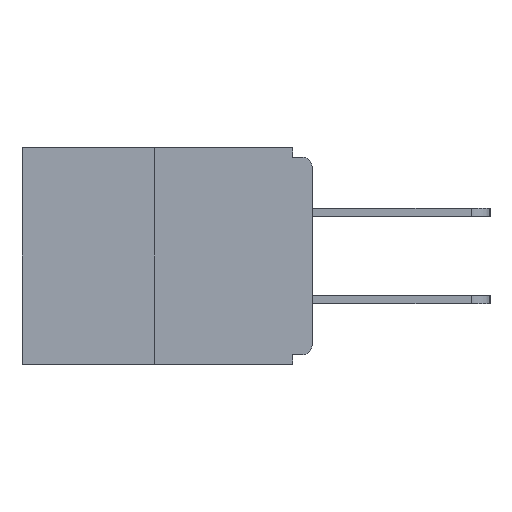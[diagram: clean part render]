
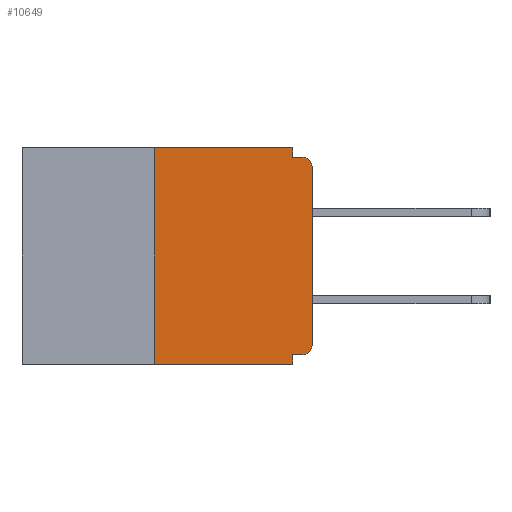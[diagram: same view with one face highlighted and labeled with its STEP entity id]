
A CAD part, left-side view. The second image highlights one B-rep face of the part: STEP entity #10649.
In plain terms, the highlighted planar face has unit normal (-1, 0, 0).
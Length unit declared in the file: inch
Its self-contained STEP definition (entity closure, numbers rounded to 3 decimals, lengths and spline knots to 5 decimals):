
#17 = CARTESIAN_POINT ( 'NONE',  ( 0., 0.015, -0.328 ) ) ;
#86 = ORIENTED_EDGE ( 'NONE', *, *, #10237, .F. ) ;
#189 = VERTEX_POINT ( 'NONE', #1568 ) ;
#205 = LINE ( 'NONE', #12582, #10612 ) ;
#230 = LINE ( 'NONE', #5191, #6545 ) ;
#375 = LINE ( 'NONE', #4759, #1457 ) ;
#461 = EDGE_CURVE ( 'NONE', #4245, #189, #2038, .T. ) ;
#812 = DIRECTION ( 'NONE',  ( 0., 0., -1. ) ) ;
#832 = DIRECTION ( 'NONE',  ( -1., 0., 0. ) ) ;
#939 = VERTEX_POINT ( 'NONE', #12508 ) ;
#1054 = DIRECTION ( 'NONE',  ( 0., -1., 0. ) ) ;
#1457 = VECTOR ( 'NONE', #12794, 39.37008 ) ;
#1568 = CARTESIAN_POINT ( 'NONE',  ( 0., 0.015, -0.015 ) ) ;
#1638 = DIRECTION ( 'NONE',  ( 0., 0., 1. ) ) ;
#1753 = CARTESIAN_POINT ( 'NONE',  ( 0., 0.015, -0.313 ) ) ;
#1868 = DIRECTION ( 'NONE',  ( 0., 1., 0. ) ) ;
#2038 = CIRCLE ( 'NONE', #5717, 0.015 ) ;
#2332 = VECTOR ( 'NONE', #4562, 39.37008 ) ;
#2425 = AXIS2_PLACEMENT_3D ( 'NONE', #1753, #832, #7921 ) ;
#2665 = ORIENTED_EDGE ( 'NONE', *, *, #10603, .T. ) ;
#2852 = LINE ( 'NONE', #7215, #5706 ) ;
#3024 = DIRECTION ( 'NONE',  ( 0., 0., -1. ) ) ;
#3090 = ORIENTED_EDGE ( 'NONE', *, *, #461, .T. ) ;
#3254 = CARTESIAN_POINT ( 'NONE',  ( 0., 0.031, 0. ) ) ;
#3560 = EDGE_CURVE ( 'NONE', #5918, #189, #230, .T. ) ;
#4131 = EDGE_CURVE ( 'NONE', #10853, #5918, #6677, .T. ) ;
#4152 = EDGE_CURVE ( 'NONE', #7958, #7381, #6830, .T. ) ;
#4245 = VERTEX_POINT ( 'NONE', #6832 ) ;
#4494 = ORIENTED_EDGE ( 'NONE', *, *, #7804, .F. ) ;
#4562 = DIRECTION ( 'NONE',  ( 0., -1., 0. ) ) ;
#4749 = EDGE_CURVE ( 'NONE', #10086, #7619, #205, .T. ) ;
#4759 = CARTESIAN_POINT ( 'NONE',  ( 0., 0.031, -0.343 ) ) ;
#4770 = VECTOR ( 'NONE', #1868, 39.37008 ) ;
#4774 = ORIENTED_EDGE ( 'NONE', *, *, #4131, .F. ) ;
#4959 = CARTESIAN_POINT ( 'NONE',  ( 0., 0.46, 0. ) ) ;
#4990 = ORIENTED_EDGE ( 'NONE', *, *, #5280, .T. ) ;
#5191 = CARTESIAN_POINT ( 'NONE',  ( 0., 0., -0.015 ) ) ;
#5280 = EDGE_CURVE ( 'NONE', #7154, #4245, #2852, .T. ) ;
#5495 = CARTESIAN_POINT ( 'NONE',  ( 0., 0.25, 0. ) ) ;
#5706 = VECTOR ( 'NONE', #6399, 39.37008 ) ;
#5717 = AXIS2_PLACEMENT_3D ( 'NONE', #8068, #11105, #3024 ) ;
#5740 = CARTESIAN_POINT ( 'NONE',  ( 0., 0., -0.313 ) ) ;
#5907 = DIRECTION ( 'NONE',  ( 0., -1., 0. ) ) ;
#5918 = VERTEX_POINT ( 'NONE', #10593 ) ;
#6399 = DIRECTION ( 'NONE',  ( 0., 0., 1. ) ) ;
#6400 = ORIENTED_EDGE ( 'NONE', *, *, #3560, .F. ) ;
#6545 = VECTOR ( 'NONE', #1054, 39.37008 ) ;
#6677 = LINE ( 'NONE', #8927, #9652 ) ;
#6830 = LINE ( 'NONE', #7773, #4770 ) ;
#6832 = CARTESIAN_POINT ( 'NONE',  ( 0., 0., -0.03 ) ) ;
#6979 = ORIENTED_EDGE ( 'NONE', *, *, #9195, .T. ) ;
#7154 = VERTEX_POINT ( 'NONE', #5740 ) ;
#7215 = CARTESIAN_POINT ( 'NONE',  ( 0., 0., 0. ) ) ;
#7381 = VERTEX_POINT ( 'NONE', #10942 ) ;
#7567 = ORIENTED_EDGE ( 'NONE', *, *, #4152, .F. ) ;
#7619 = VERTEX_POINT ( 'NONE', #5495 ) ;
#7773 = CARTESIAN_POINT ( 'NONE',  ( 0., 0., -0.328 ) ) ;
#7804 = EDGE_CURVE ( 'NONE', #7381, #939, #375, .T. ) ;
#7921 = DIRECTION ( 'NONE',  ( 0., 0., -1. ) ) ;
#7958 = VERTEX_POINT ( 'NONE', #17 ) ;
#8068 = CARTESIAN_POINT ( 'NONE',  ( 0., 0.015, -0.03 ) ) ;
#8624 = PLANE ( 'NONE',  #9605 ) ;
#8751 = CARTESIAN_POINT ( 'NONE',  ( 0., 0.46, 0. ) ) ;
#8927 = CARTESIAN_POINT ( 'NONE',  ( 0., 0.031, 0. ) ) ;
#9195 = EDGE_CURVE ( 'NONE', #7958, #7154, #11684, .T. ) ;
#9605 = AXIS2_PLACEMENT_3D ( 'NONE', #8751, #12850, #812 ) ;
#9652 = VECTOR ( 'NONE', #9924, 39.37008 ) ;
#9727 = LINE ( 'NONE', #10604, #2332 ) ;
#9924 = DIRECTION ( 'NONE',  ( 0., 0., -1. ) ) ;
#10086 = VERTEX_POINT ( 'NONE', #11809 ) ;
#10237 = EDGE_CURVE ( 'NONE', #7619, #10853, #11814, .T. ) ;
#10593 = CARTESIAN_POINT ( 'NONE',  ( 0., 0.031, -0.015 ) ) ;
#10603 = EDGE_CURVE ( 'NONE', #10086, #939, #9727, .T. ) ;
#10604 = CARTESIAN_POINT ( 'NONE',  ( 0., 0.46, -0.343 ) ) ;
#10612 = VECTOR ( 'NONE', #1638, 39.37008 ) ;
#10649 = ADVANCED_FACE ( 'NONE', ( #12432 ), #8624, .F. ) ;
#10853 = VERTEX_POINT ( 'NONE', #3254 ) ;
#10942 = CARTESIAN_POINT ( 'NONE',  ( 0., 0.031, -0.328 ) ) ;
#11038 = ORIENTED_EDGE ( 'NONE', *, *, #4749, .F. ) ;
#11105 = DIRECTION ( 'NONE',  ( -1., 0., 0. ) ) ;
#11654 = VECTOR ( 'NONE', #5907, 39.37008 ) ;
#11684 = CIRCLE ( 'NONE', #2425, 0.015 ) ;
#11809 = CARTESIAN_POINT ( 'NONE',  ( 0., 0.25, -0.343 ) ) ;
#11814 = LINE ( 'NONE', #4959, #11654 ) ;
#12432 = FACE_OUTER_BOUND ( 'NONE', #12488, .T. ) ;
#12488 = EDGE_LOOP ( 'NONE', ( #86, #11038, #2665, #4494, #7567, #6979, #4990, #3090, #6400, #4774 ) ) ;
#12508 = CARTESIAN_POINT ( 'NONE',  ( 0., 0.031, -0.343 ) ) ;
#12582 = CARTESIAN_POINT ( 'NONE',  ( 0., 0.25, 0. ) ) ;
#12794 = DIRECTION ( 'NONE',  ( 0., 0., -1. ) ) ;
#12850 = DIRECTION ( 'NONE',  ( 1., 0., 0. ) ) ;
